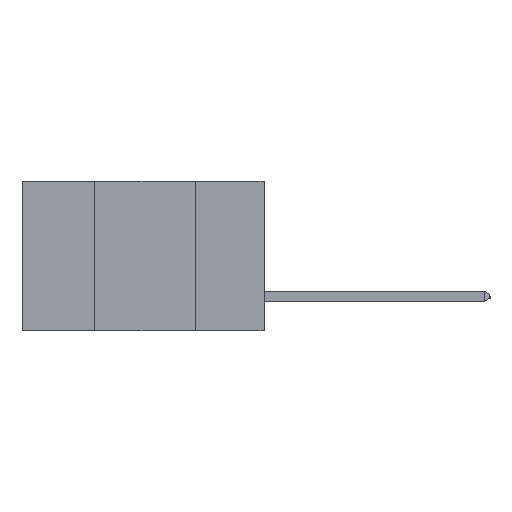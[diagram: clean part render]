
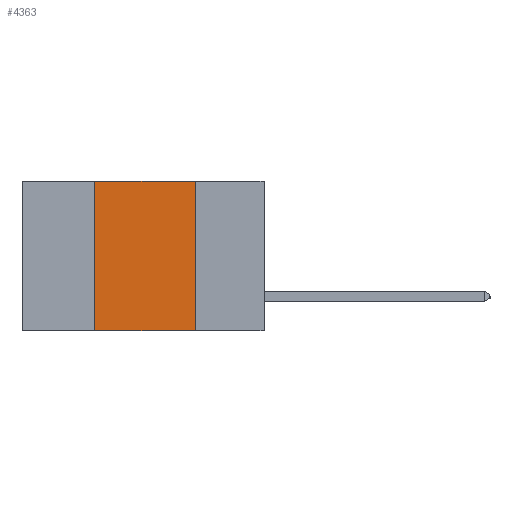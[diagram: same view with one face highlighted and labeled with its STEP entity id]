
A CAD part, left-side view. The second image highlights one B-rep face of the part: STEP entity #4363.
In plain terms, the highlighted planar face has unit normal (-1, 0, 0).
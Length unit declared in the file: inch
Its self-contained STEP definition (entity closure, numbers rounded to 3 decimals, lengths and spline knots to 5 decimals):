
#1168 = ORIENTED_EDGE ( 'NONE', *, *, #17990, .T. ) ;
#1374 = VERTEX_POINT ( 'NONE', #1690 ) ;
#1690 = CARTESIAN_POINT ( 'NONE',  ( 0., 0.17, -0.37 ) ) ;
#1878 = VECTOR ( 'NONE', #2631, 39.37008 ) ;
#2631 = DIRECTION ( 'NONE',  ( 0., 0., -1. ) ) ;
#4363 = ADVANCED_FACE ( 'NONE', ( #17418 ), #4865, .F. ) ;
#4440 = ORIENTED_EDGE ( 'NONE', *, *, #11052, .F. ) ;
#4733 = EDGE_CURVE ( 'NONE', #10787, #15117, #9541, .T. ) ;
#4827 = DIRECTION ( 'NONE',  ( 0., 0., 1. ) ) ;
#4834 = DIRECTION ( 'NONE',  ( 1., 0., 0. ) ) ;
#4865 = PLANE ( 'NONE',  #22802 ) ;
#5517 = CARTESIAN_POINT ( 'NONE',  ( 0., 0.6, 0. ) ) ;
#6913 = DIRECTION ( 'NONE',  ( 0., -1., 0. ) ) ;
#7168 = CARTESIAN_POINT ( 'NONE',  ( 0., 0.17, 0. ) ) ;
#7680 = EDGE_LOOP ( 'NONE', ( #12619, #22342, #4440, #1168 ) ) ;
#9541 = LINE ( 'NONE', #20058, #13863 ) ;
#9576 = CARTESIAN_POINT ( 'NONE',  ( 0., 0.42, 0. ) ) ;
#10332 = LINE ( 'NONE', #15820, #19745 ) ;
#10692 = VERTEX_POINT ( 'NONE', #18323 ) ;
#10787 = VERTEX_POINT ( 'NONE', #9576 ) ;
#10998 = DIRECTION ( 'NONE',  ( 0., 0., -1. ) ) ;
#11052 = EDGE_CURVE ( 'NONE', #10692, #10787, #10332, .T. ) ;
#11666 = VECTOR ( 'NONE', #6913, 39.37008 ) ;
#12619 = ORIENTED_EDGE ( 'NONE', *, *, #16195, .F. ) ;
#13863 = VECTOR ( 'NONE', #17310, 39.37008 ) ;
#15117 = VERTEX_POINT ( 'NONE', #7168 ) ;
#15820 = CARTESIAN_POINT ( 'NONE',  ( 0., 0.42, 0. ) ) ;
#16195 = EDGE_CURVE ( 'NONE', #15117, #1374, #21130, .T. ) ;
#17310 = DIRECTION ( 'NONE',  ( 0., -1., 0. ) ) ;
#17327 = CARTESIAN_POINT ( 'NONE',  ( 0., 0.17, 0. ) ) ;
#17418 = FACE_OUTER_BOUND ( 'NONE', #7680, .T. ) ;
#17990 = EDGE_CURVE ( 'NONE', #10692, #1374, #20412, .T. ) ;
#18323 = CARTESIAN_POINT ( 'NONE',  ( 0., 0.42, -0.37 ) ) ;
#19459 = CARTESIAN_POINT ( 'NONE',  ( 0., 0.6, -0.37 ) ) ;
#19745 = VECTOR ( 'NONE', #4827, 39.37008 ) ;
#20058 = CARTESIAN_POINT ( 'NONE',  ( 0., 0.6, 0. ) ) ;
#20412 = LINE ( 'NONE', #19459, #11666 ) ;
#21130 = LINE ( 'NONE', #17327, #1878 ) ;
#22342 = ORIENTED_EDGE ( 'NONE', *, *, #4733, .F. ) ;
#22802 = AXIS2_PLACEMENT_3D ( 'NONE', #5517, #4834, #10998 ) ;
